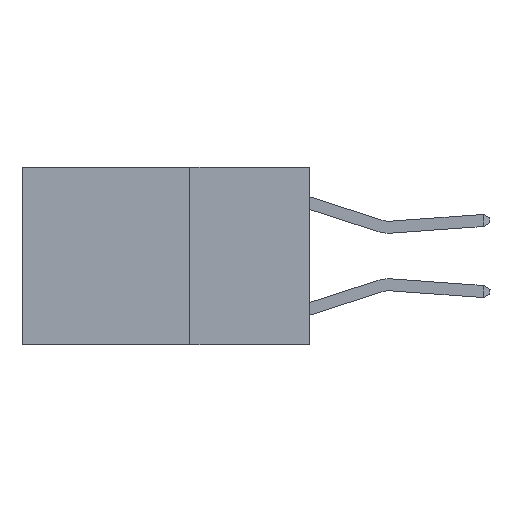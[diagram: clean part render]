
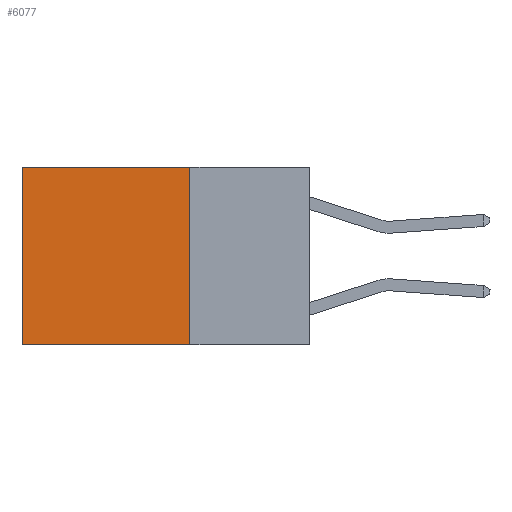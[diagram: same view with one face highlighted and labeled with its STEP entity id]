
A CAD part, left-side view. The second image highlights one B-rep face of the part: STEP entity #6077.
In plain terms, the highlighted planar face has unit normal (-1, 0, 0).
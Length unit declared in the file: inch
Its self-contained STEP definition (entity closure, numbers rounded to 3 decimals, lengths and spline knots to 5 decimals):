
#5 = EDGE_CURVE ( 'NONE', #6050, #10016, #3699, .T. ) ;
#491 = AXIS2_PLACEMENT_3D ( 'NONE', #9795, #7466, #2524 ) ;
#1108 = EDGE_CURVE ( 'NONE', #10016, #2393, #6242, .T. ) ;
#1140 = DIRECTION ( 'NONE',  ( 0., 1., 0. ) ) ;
#1451 = VECTOR ( 'NONE', #4033, 39.37008 ) ;
#1575 = ORIENTED_EDGE ( 'NONE', *, *, #10464, .T. ) ;
#1605 = CARTESIAN_POINT ( 'NONE',  ( 0.2625, 0.6, -0.37 ) ) ;
#1662 = PLANE ( 'NONE',  #491 ) ;
#1993 = CARTESIAN_POINT ( 'NONE',  ( 0.2625, 0.25, 0. ) ) ;
#2142 = VERTEX_POINT ( 'NONE', #7889 ) ;
#2393 = VERTEX_POINT ( 'NONE', #1605 ) ;
#2450 = CARTESIAN_POINT ( 'NONE',  ( 0.2625, 0.25, 0. ) ) ;
#2524 = DIRECTION ( 'NONE',  ( 0., 0., -1. ) ) ;
#2965 = CARTESIAN_POINT ( 'NONE',  ( 0.2625, 0.25, -0.37 ) ) ;
#3699 = LINE ( 'NONE', #6651, #1451 ) ;
#3700 = LINE ( 'NONE', #1993, #8029 ) ;
#4033 = DIRECTION ( 'NONE',  ( 0., 0., -1. ) ) ;
#4954 = ORIENTED_EDGE ( 'NONE', *, *, #1108, .F. ) ;
#5265 = DIRECTION ( 'NONE',  ( 0., 0., -1. ) ) ;
#5999 = LINE ( 'NONE', #10055, #8383 ) ;
#6050 = VERTEX_POINT ( 'NONE', #2450 ) ;
#6077 = ADVANCED_FACE ( 'NONE', ( #8450 ), #1662, .F. ) ;
#6242 = LINE ( 'NONE', #7845, #6511 ) ;
#6511 = VECTOR ( 'NONE', #1140, 39.37008 ) ;
#6514 = ORIENTED_EDGE ( 'NONE', *, *, #5, .F. ) ;
#6651 = CARTESIAN_POINT ( 'NONE',  ( 0.2625, 0.25, 0. ) ) ;
#7179 = EDGE_LOOP ( 'NONE', ( #1575, #4954, #6514, #9623 ) ) ;
#7466 = DIRECTION ( 'NONE',  ( 1., 0., 0. ) ) ;
#7845 = CARTESIAN_POINT ( 'NONE',  ( 0.2625, 0.25, -0.37 ) ) ;
#7889 = CARTESIAN_POINT ( 'NONE',  ( 0.2625, 0.6, 0. ) ) ;
#8029 = VECTOR ( 'NONE', #8545, 39.37008 ) ;
#8383 = VECTOR ( 'NONE', #5265, 39.37008 ) ;
#8450 = FACE_OUTER_BOUND ( 'NONE', #7179, .T. ) ;
#8545 = DIRECTION ( 'NONE',  ( 0., 1., 0. ) ) ;
#9623 = ORIENTED_EDGE ( 'NONE', *, *, #9875, .T. ) ;
#9795 = CARTESIAN_POINT ( 'NONE',  ( 0.2625, 0.25, 0. ) ) ;
#9875 = EDGE_CURVE ( 'NONE', #6050, #2142, #3700, .T. ) ;
#10016 = VERTEX_POINT ( 'NONE', #2965 ) ;
#10055 = CARTESIAN_POINT ( 'NONE',  ( 0.2625, 0.6, 0. ) ) ;
#10464 = EDGE_CURVE ( 'NONE', #2142, #2393, #5999, .T. ) ;
